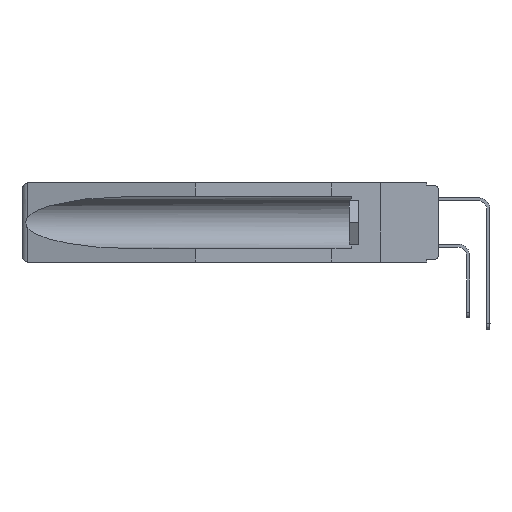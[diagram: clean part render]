
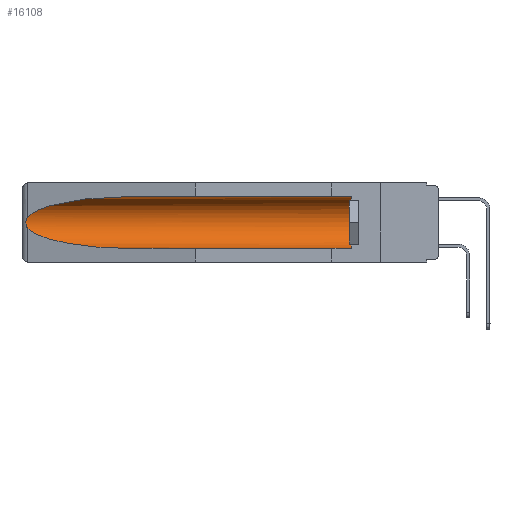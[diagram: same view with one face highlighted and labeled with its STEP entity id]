
A CAD part, left-side view. The second image highlights one B-rep face of the part: STEP entity #16108.
In plain terms, the highlighted cylindrical face has radius 2.857 mm (diameter 5.715 mm), a partial arc.
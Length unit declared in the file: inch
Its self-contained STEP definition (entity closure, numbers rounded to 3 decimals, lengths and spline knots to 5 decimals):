
#28 = ORIENTED_EDGE ( 'NONE', *, *, #17946, .T. ) ;
#1886 = CARTESIAN_POINT ( 'NONE',  ( 0.155, 0.126, -0.284 ) ) ;
#1997 = CARTESIAN_POINT ( 'NONE',  ( 0.155, -0.30754, -0.059 ) ) ;
#2247 = CARTESIAN_POINT ( 'NONE',  ( 0.25451, 1.48313, -0.24835 ) ) ;
#3357 = VECTOR ( 'NONE', #17590, 39.37008 ) ;
#3527 = LINE ( 'NONE', #1997, #18041 ) ;
#3634 = ORIENTED_EDGE ( 'NONE', *, *, #4501, .T. ) ;
#4332 = CARTESIAN_POINT ( 'NONE',  ( 0.26537, 1.52718, -0.14972 ) ) ;
#4424 = CARTESIAN_POINT ( 'NONE',  ( 0.21114, 1.30732, -0.059 ) ) ;
#4501 = EDGE_CURVE ( 'NONE', #17665, #10720, #12070, .T. ) ;
#4636 = VERTEX_POINT ( 'NONE', #1886 ) ;
#4697 = CYLINDRICAL_SURFACE ( 'NONE', #11222, 0.1125 ) ;
#5169 = CARTESIAN_POINT ( 'NONE',  ( 0.26537, 1.52718, -0.14972 ) ) ;
#5262 = CARTESIAN_POINT ( 'NONE',  ( 0.2675, 1.53308, -0.16763 ) ) ;
#5443 = CARTESIAN_POINT ( 'NONE',  ( 0.155, 0.126, -0.059 ) ) ;
#5584 = DIRECTION ( 'NONE',  ( 0., -1., 0. ) ) ;
#5898 = CARTESIAN_POINT ( 'NONE',  ( 0.26537, 1.52718, -0.19328 ) ) ;
#6400 = DIRECTION ( 'NONE',  ( 0., 0., 1. ) ) ;
#6503 = CIRCLE ( 'NONE', #9716, 0.1125 ) ;
#6573 = CARTESIAN_POINT ( 'NONE',  ( 0.2673, 1.53269, -0.17917 ) ) ;
#6777 = CARTESIAN_POINT ( 'NONE',  ( 0.26537, 1.52718, -0.19328 ) ) ;
#6804 =( BOUNDED_CURVE ( )  B_SPLINE_CURVE ( 3, ( #6777, #2247, #11277, #17304 ),
 .UNSPECIFIED., .F., .T. ) 
 B_SPLINE_CURVE_WITH_KNOTS ( ( 4, 4 ),
 ( 0.1948, 1.5708 ),
 .UNSPECIFIED. ) 
 CURVE ( )  GEOMETRIC_REPRESENTATION_ITEM ( )  RATIONAL_B_SPLINE_CURVE ( ( 1., 0.848, 0.848, 1. ) ) 
 REPRESENTATION_ITEM ( '' )  );
#6873 = CARTESIAN_POINT ( 'NONE',  ( 0.26655, 1.53094, -0.18657 ) ) ;
#7034 = EDGE_CURVE ( 'NONE', #7457, #13670, #6804, .T. ) ;
#7457 = VERTEX_POINT ( 'NONE', #5898 ) ;
#8016 = FACE_OUTER_BOUND ( 'NONE', #15510, .T. ) ;
#8136 = DIRECTION ( 'NONE',  ( 0., 1., 0. ) ) ;
#8602 = CARTESIAN_POINT ( 'NONE',  ( 0.155, 1.07973, -0.284 ) ) ;
#8633 = CARTESIAN_POINT ( 'NONE',  ( 0.26537, 1.52718, -0.14972 ) ) ;
#8961 = ORIENTED_EDGE ( 'NONE', *, *, #12048, .T. ) ;
#9205 = CARTESIAN_POINT ( 'NONE',  ( 0.155, 1.07973, -0.059 ) ) ;
#9228 = CARTESIAN_POINT ( 'NONE',  ( 0.155, 1.07973, -0.059 ) ) ;
#9241 = ORIENTED_EDGE ( 'NONE', *, *, #19712, .F. ) ;
#9716 = AXIS2_PLACEMENT_3D ( 'NONE', #11397, #5584, #14813 ) ;
#9870 = CARTESIAN_POINT ( 'NONE',  ( 0.26597, 1.52961, -0.15275 ) ) ;
#10255 = VERTEX_POINT ( 'NONE', #5443 ) ;
#10720 = VERTEX_POINT ( 'NONE', #8633 ) ;
#10804 = CARTESIAN_POINT ( 'NONE',  ( 0.155, -0.30754, -0.1715 ) ) ;
#11222 = AXIS2_PLACEMENT_3D ( 'NONE', #10804, #15536, #6400 ) ;
#11277 = CARTESIAN_POINT ( 'NONE',  ( 0.21114, 1.30732, -0.284 ) ) ;
#11397 = CARTESIAN_POINT ( 'NONE',  ( 0.155, 0.126, -0.1715 ) ) ;
#11858 = CARTESIAN_POINT ( 'NONE',  ( 0.26654, 1.53092, -0.15636 ) ) ;
#12048 = EDGE_CURVE ( 'NONE', #10255, #17665, #3527, .T. ) ;
#12070 =( BOUNDED_CURVE ( )  B_SPLINE_CURVE ( 3, ( #9228, #4424, #19449, #4332 ),
 .UNSPECIFIED., .F., .T. ) 
 B_SPLINE_CURVE_WITH_KNOTS ( ( 4, 4 ),
 ( 4.71239, 6.08839 ),
 .UNSPECIFIED. ) 
 CURVE ( )  GEOMETRIC_REPRESENTATION_ITEM ( )  RATIONAL_B_SPLINE_CURVE ( ( 1., 0.848, 0.848, 1. ) ) 
 REPRESENTATION_ITEM ( '' )  );
#13670 = VERTEX_POINT ( 'NONE', #8602 ) ;
#14813 = DIRECTION ( 'NONE',  ( 0., 0., 1. ) ) ;
#14836 = ORIENTED_EDGE ( 'NONE', *, *, #7034, .T. ) ;
#15510 = EDGE_LOOP ( 'NONE', ( #3634, #19514, #14836, #9241, #28, #8961 ) ) ;
#15536 = DIRECTION ( 'NONE',  ( 0., 1., 0. ) ) ;
#15893 = CARTESIAN_POINT ( 'NONE',  ( 0.26537, 1.52718, -0.19328 ) ) ;
#16108 = ADVANCED_FACE ( 'NONE', ( #8016 ), #4697, .F. ) ;
#16202 = LINE ( 'NONE', #19083, #3357 ) ;
#16460 = CARTESIAN_POINT ( 'NONE',  ( 0.2675, 1.53308, -0.17534 ) ) ;
#16508 = B_SPLINE_CURVE_WITH_KNOTS ( 'NONE', 3,
 ( #5169, #9870, #11858, #18977, #5262, #16460, #6573, #6873, #18785, #15893 ),
 .UNSPECIFIED., .F., .F.,
 ( 4, 2, 2, 2, 4 ),
 ( 0., 0.00029, 0.00058, 0.00087, 0.00117 ),
 .UNSPECIFIED. ) ;
#17075 = EDGE_CURVE ( 'NONE', #10720, #7457, #16508, .T. ) ;
#17304 = CARTESIAN_POINT ( 'NONE',  ( 0.155, 1.07973, -0.284 ) ) ;
#17590 = DIRECTION ( 'NONE',  ( 0., 1., 0. ) ) ;
#17665 = VERTEX_POINT ( 'NONE', #9205 ) ;
#17946 = EDGE_CURVE ( 'NONE', #4636, #10255, #6503, .T. ) ;
#18041 = VECTOR ( 'NONE', #8136, 39.37008 ) ;
#18785 = CARTESIAN_POINT ( 'NONE',  ( 0.26597, 1.5296, -0.19026 ) ) ;
#18977 = CARTESIAN_POINT ( 'NONE',  ( 0.2673, 1.5327, -0.16383 ) ) ;
#19083 = CARTESIAN_POINT ( 'NONE',  ( 0.155, -0.30754, -0.284 ) ) ;
#19449 = CARTESIAN_POINT ( 'NONE',  ( 0.25451, 1.48313, -0.09465 ) ) ;
#19514 = ORIENTED_EDGE ( 'NONE', *, *, #17075, .T. ) ;
#19712 = EDGE_CURVE ( 'NONE', #4636, #13670, #16202, .T. ) ;
